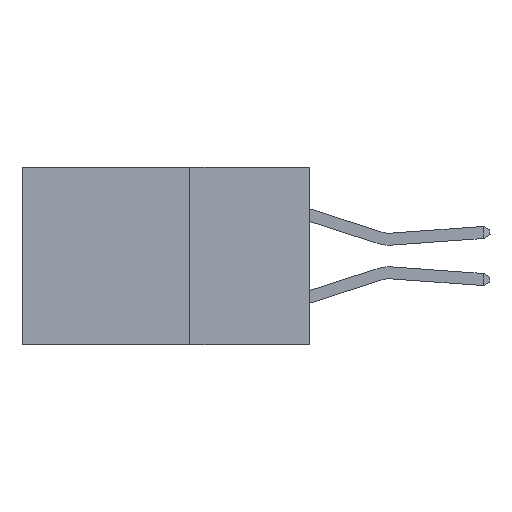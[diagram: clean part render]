
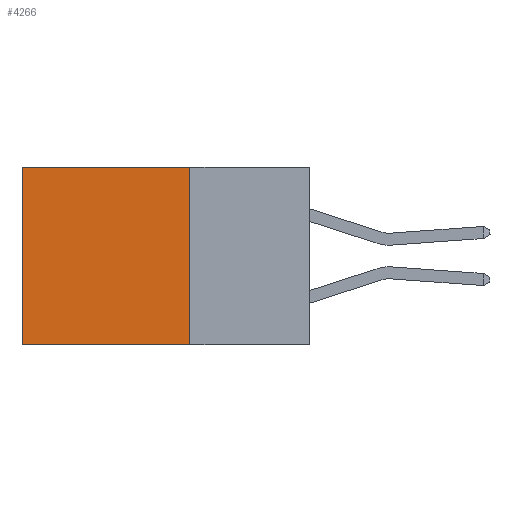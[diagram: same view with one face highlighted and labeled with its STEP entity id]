
A CAD part, left-side view. The second image highlights one B-rep face of the part: STEP entity #4266.
In plain terms, the highlighted planar face has unit normal (-1, 0, 0).
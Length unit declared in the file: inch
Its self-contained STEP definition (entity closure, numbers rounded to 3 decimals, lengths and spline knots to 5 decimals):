
#205 = PLANE ( 'NONE',  #2967 ) ;
#289 = CARTESIAN_POINT ( 'NONE',  ( 0.298, 0.6, 0. ) ) ;
#431 = FACE_OUTER_BOUND ( 'NONE', #4066, .T. ) ;
#1536 = CARTESIAN_POINT ( 'NONE',  ( 0.298, 0.25, -0.37 ) ) ;
#1883 = CARTESIAN_POINT ( 'NONE',  ( 0.298, 0.6, 0. ) ) ;
#2503 = EDGE_CURVE ( 'NONE', #6203, #5846, #5610, .T. ) ;
#2690 = EDGE_CURVE ( 'NONE', #5846, #3773, #3838, .T. ) ;
#2770 = DIRECTION ( 'NONE',  ( 1., 0., 0. ) ) ;
#2967 = AXIS2_PLACEMENT_3D ( 'NONE', #4634, #2770, #5362 ) ;
#3773 = VERTEX_POINT ( 'NONE', #10205 ) ;
#3838 = LINE ( 'NONE', #289, #7539 ) ;
#4066 = EDGE_LOOP ( 'NONE', ( #9986, #10475, #8191, #4440 ) ) ;
#4266 = ADVANCED_FACE ( 'NONE', ( #431 ), #205, .F. ) ;
#4440 = ORIENTED_EDGE ( 'NONE', *, *, #2503, .T. ) ;
#4605 = DIRECTION ( 'NONE',  ( 0., 0., -1. ) ) ;
#4634 = CARTESIAN_POINT ( 'NONE',  ( 0.298, 0.25, 0. ) ) ;
#5029 = DIRECTION ( 'NONE',  ( 0., 1., 0. ) ) ;
#5138 = CARTESIAN_POINT ( 'NONE',  ( 0.298, 0.25, -0.37 ) ) ;
#5310 = DIRECTION ( 'NONE',  ( 0., 1., 0. ) ) ;
#5362 = DIRECTION ( 'NONE',  ( 0., 0., -1. ) ) ;
#5369 = LINE ( 'NONE', #1536, #7695 ) ;
#5610 = LINE ( 'NONE', #10596, #10070 ) ;
#5846 = VERTEX_POINT ( 'NONE', #1883 ) ;
#6035 = EDGE_CURVE ( 'NONE', #6203, #7923, #8448, .T. ) ;
#6203 = VERTEX_POINT ( 'NONE', #7054 ) ;
#6509 = DIRECTION ( 'NONE',  ( 0., 0., -1. ) ) ;
#6548 = CARTESIAN_POINT ( 'NONE',  ( 0.298, 0.25, 0. ) ) ;
#6919 = VECTOR ( 'NONE', #6509, 39.37008 ) ;
#7054 = CARTESIAN_POINT ( 'NONE',  ( 0.298, 0.25, 0. ) ) ;
#7539 = VECTOR ( 'NONE', #4605, 39.37008 ) ;
#7662 = EDGE_CURVE ( 'NONE', #7923, #3773, #5369, .T. ) ;
#7695 = VECTOR ( 'NONE', #5029, 39.37008 ) ;
#7923 = VERTEX_POINT ( 'NONE', #5138 ) ;
#8191 = ORIENTED_EDGE ( 'NONE', *, *, #6035, .F. ) ;
#8448 = LINE ( 'NONE', #6548, #6919 ) ;
#9986 = ORIENTED_EDGE ( 'NONE', *, *, #2690, .T. ) ;
#10070 = VECTOR ( 'NONE', #5310, 39.37008 ) ;
#10205 = CARTESIAN_POINT ( 'NONE',  ( 0.298, 0.6, -0.37 ) ) ;
#10475 = ORIENTED_EDGE ( 'NONE', *, *, #7662, .F. ) ;
#10596 = CARTESIAN_POINT ( 'NONE',  ( 0.298, 0.25, 0. ) ) ;
